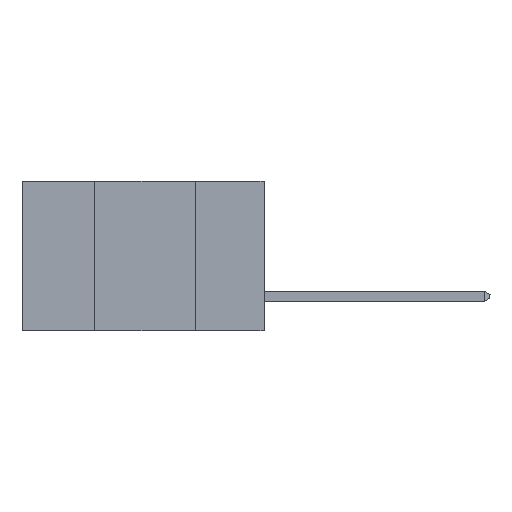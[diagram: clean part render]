
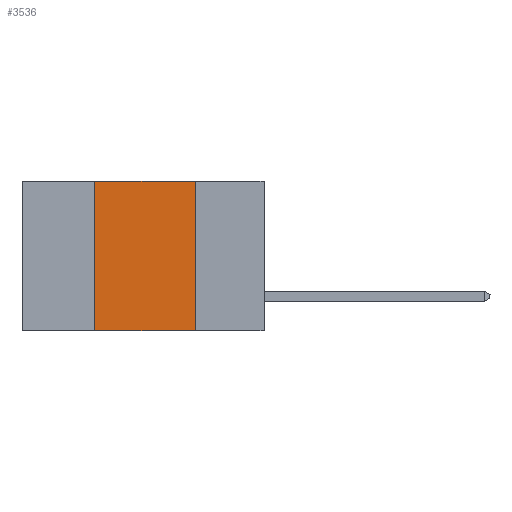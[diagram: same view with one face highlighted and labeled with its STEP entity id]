
A CAD part, left-side view. The second image highlights one B-rep face of the part: STEP entity #3536.
In plain terms, the highlighted planar face has unit normal (-1, 0, 0).
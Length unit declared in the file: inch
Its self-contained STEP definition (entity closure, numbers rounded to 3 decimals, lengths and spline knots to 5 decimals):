
#31 = CARTESIAN_POINT ( 'NONE',  ( 0., 0.42, 0. ) ) ;
#588 = AXIS2_PLACEMENT_3D ( 'NONE', #2431, #18254, #9288 ) ;
#729 = CARTESIAN_POINT ( 'NONE',  ( 0., 0.17, -0.37 ) ) ;
#2012 = CARTESIAN_POINT ( 'NONE',  ( 0., 0.6, 0. ) ) ;
#2297 = LINE ( 'NONE', #20089, #15898 ) ;
#2357 = ORIENTED_EDGE ( 'NONE', *, *, #18048, .F. ) ;
#2431 = CARTESIAN_POINT ( 'NONE',  ( 0., 0.6, 0. ) ) ;
#2517 = EDGE_CURVE ( 'NONE', #13460, #15000, #14109, .T. ) ;
#2730 = CARTESIAN_POINT ( 'NONE',  ( 0., 0.42, -0.37 ) ) ;
#3536 = ADVANCED_FACE ( 'NONE', ( #11131 ), #12771, .F. ) ;
#5011 = CARTESIAN_POINT ( 'NONE',  ( 0., 0.17, -0.37 ) ) ;
#5463 = EDGE_CURVE ( 'NONE', #18881, #8198, #2297, .T. ) ;
#7935 = CARTESIAN_POINT ( 'NONE',  ( 0., 0.42, -0.37 ) ) ;
#7950 = ORIENTED_EDGE ( 'NONE', *, *, #16855, .F. ) ;
#7954 = VECTOR ( 'NONE', #10457, 39.37008 ) ;
#8198 = VERTEX_POINT ( 'NONE', #729 ) ;
#9288 = DIRECTION ( 'NONE',  ( 0., 0., -1. ) ) ;
#10457 = DIRECTION ( 'NONE',  ( 0., 0., -1. ) ) ;
#10539 = VECTOR ( 'NONE', #12832, 39.37008 ) ;
#11131 = FACE_OUTER_BOUND ( 'NONE', #19636, .T. ) ;
#12771 = PLANE ( 'NONE',  #588 ) ;
#12832 = DIRECTION ( 'NONE',  ( 0., -1., 0. ) ) ;
#13405 = CARTESIAN_POINT ( 'NONE',  ( 0., 0.17, 0. ) ) ;
#13460 = VERTEX_POINT ( 'NONE', #31 ) ;
#14109 = LINE ( 'NONE', #2012, #10539 ) ;
#14977 = DIRECTION ( 'NONE',  ( 0., -1., 0. ) ) ;
#15000 = VERTEX_POINT ( 'NONE', #13405 ) ;
#15898 = VECTOR ( 'NONE', #14977, 39.37008 ) ;
#16855 = EDGE_CURVE ( 'NONE', #15000, #8198, #20824, .T. ) ;
#18048 = EDGE_CURVE ( 'NONE', #18881, #13460, #22039, .T. ) ;
#18254 = DIRECTION ( 'NONE',  ( 1., 0., 0. ) ) ;
#18464 = DIRECTION ( 'NONE',  ( 0., 0., 1. ) ) ;
#18881 = VERTEX_POINT ( 'NONE', #7935 ) ;
#18929 = ORIENTED_EDGE ( 'NONE', *, *, #5463, .T. ) ;
#19636 = EDGE_LOOP ( 'NONE', ( #7950, #21199, #2357, #18929 ) ) ;
#20089 = CARTESIAN_POINT ( 'NONE',  ( 0., 0.6, -0.37 ) ) ;
#20590 = VECTOR ( 'NONE', #18464, 39.37008 ) ;
#20824 = LINE ( 'NONE', #5011, #7954 ) ;
#21199 = ORIENTED_EDGE ( 'NONE', *, *, #2517, .F. ) ;
#22039 = LINE ( 'NONE', #2730, #20590 ) ;
